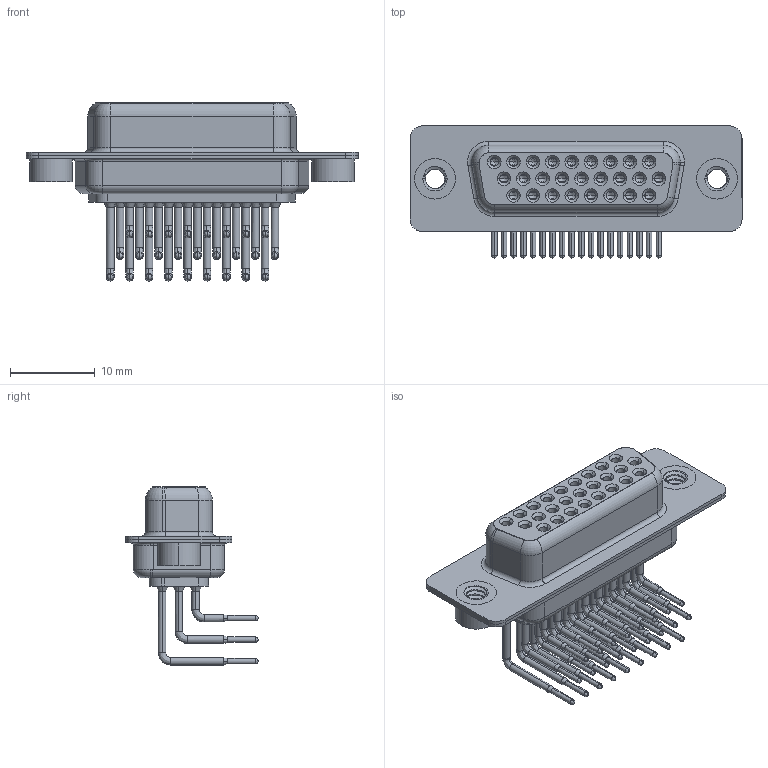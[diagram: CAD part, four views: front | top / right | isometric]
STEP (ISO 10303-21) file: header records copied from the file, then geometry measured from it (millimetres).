
FILE_DESCRIPTION (( 'STEP AP203' ), '1' );
FILE_NAME ('634-M26-663-WT2.STEP', '2018-09-28T00:02:52', ( '' ), ( '' ), 'SwSTEP 2.0', 'SolidWorks 2016', '' );
FILE_SCHEMA (( 'CONFIG_CONTROL_DESIGN' ));
Length unit declared in the file: millimetre
Products named in the file (8): 634M Contact Row 3; 634M 4-40 Threaded Rivet; 634-M26-663-WT2; 634M Housing_26 Contacts; 634M Shell Front_26 Contacts; 634M Shell Rear_26 Contacts; 634M Contact Row 1; 634M Contact Row 2
Assembly tree (31 placements, depth 2):
  634-M26-663-WT2
    634M Housing_26 Contacts
    634M Shell Front_26 Contacts
    634M Shell Rear_26 Contacts
    634M Contact Row 1  x9
    634M Contact Row 2  x9
    634M Contact Row 3  x8
    634M 4-40 Threaded Rivet  x2
Bounding box: 39.2 x 15.6 x 21.02 mm (x, y, z)
Volume: 2532.9 mm3; surface area: 8471.4 mm2
Topology: 31 solids, 31 shells, 1657 faces, 4197 edges, 2639 vertices
Faces by surface type: cylinder 735, plane 457, cone 292, bspline 110, torus 63
Entity records: 23743 total; most frequent: CARTESIAN_POINT 5363, DIRECTION 3893, ORIENTED_EDGE 3284, EDGE_CURVE 1642, AXIS2_PLACEMENT_3D 1631, VERTEX_POINT 1045, CIRCLE 908, EDGE_LOOP 863
